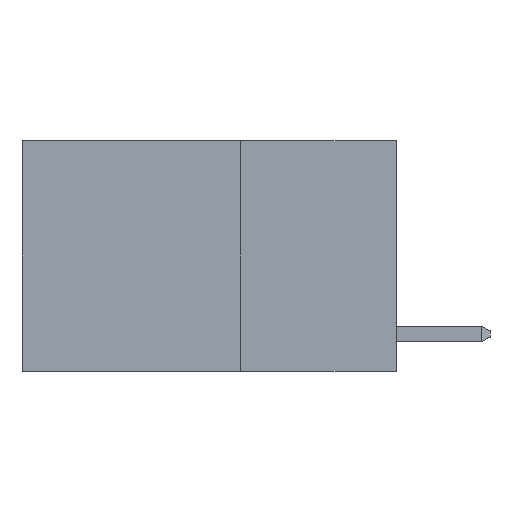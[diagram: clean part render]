
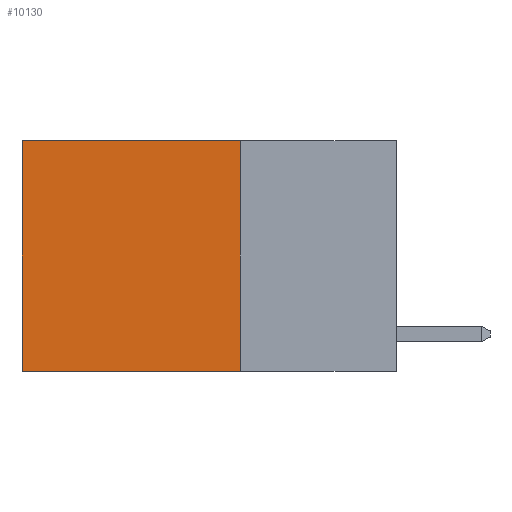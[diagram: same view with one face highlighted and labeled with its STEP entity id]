
A CAD part, left-side view. The second image highlights one B-rep face of the part: STEP entity #10130.
In plain terms, the highlighted planar face has unit normal (-1, 0, 0).
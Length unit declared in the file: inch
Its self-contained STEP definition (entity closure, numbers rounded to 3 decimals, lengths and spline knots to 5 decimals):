
#72 = DIRECTION ( 'NONE',  ( 0., 1., 0. ) ) ;
#144 = AXIS2_PLACEMENT_3D ( 'NONE', #7745, #2744, #8549 ) ;
#897 = VECTOR ( 'NONE', #9569, 39.37008 ) ;
#1374 = LINE ( 'NONE', #5203, #10183 ) ;
#1540 = CARTESIAN_POINT ( 'NONE',  ( 0.2625, 0.25, 0. ) ) ;
#1907 = CARTESIAN_POINT ( 'NONE',  ( 0.2625, 0.6, -0.37 ) ) ;
#2203 = VERTEX_POINT ( 'NONE', #8564 ) ;
#2212 = EDGE_CURVE ( 'NONE', #9869, #2259, #6010, .T. ) ;
#2259 = VERTEX_POINT ( 'NONE', #10237 ) ;
#2744 = DIRECTION ( 'NONE',  ( 1., 0., 0. ) ) ;
#3864 = CARTESIAN_POINT ( 'NONE',  ( 0.2625, 0.25, 0. ) ) ;
#4023 = VECTOR ( 'NONE', #6157, 39.37008 ) ;
#4359 = LINE ( 'NONE', #4698, #897 ) ;
#4404 = PLANE ( 'NONE',  #144 ) ;
#4698 = CARTESIAN_POINT ( 'NONE',  ( 0.2625, 0.6, 0. ) ) ;
#5197 = ORIENTED_EDGE ( 'NONE', *, *, #2212, .T. ) ;
#5203 = CARTESIAN_POINT ( 'NONE',  ( 0.2625, 0.25, -0.37 ) ) ;
#5490 = EDGE_CURVE ( 'NONE', #9869, #2203, #10479, .T. ) ;
#5571 = ORIENTED_EDGE ( 'NONE', *, *, #7923, .F. ) ;
#6010 = LINE ( 'NONE', #10158, #4023 ) ;
#6157 = DIRECTION ( 'NONE',  ( 0., 1., 0. ) ) ;
#6208 = VECTOR ( 'NONE', #8789, 39.37008 ) ;
#6832 = FACE_OUTER_BOUND ( 'NONE', #9192, .T. ) ;
#7659 = ORIENTED_EDGE ( 'NONE', *, *, #9658, .T. ) ;
#7745 = CARTESIAN_POINT ( 'NONE',  ( 0.2625, 0.25, 0. ) ) ;
#7923 = EDGE_CURVE ( 'NONE', #2203, #10164, #1374, .T. ) ;
#8549 = DIRECTION ( 'NONE',  ( 0., 0., -1. ) ) ;
#8564 = CARTESIAN_POINT ( 'NONE',  ( 0.2625, 0.25, -0.37 ) ) ;
#8789 = DIRECTION ( 'NONE',  ( 0., 0., -1. ) ) ;
#9192 = EDGE_LOOP ( 'NONE', ( #7659, #5571, #9690, #5197 ) ) ;
#9569 = DIRECTION ( 'NONE',  ( 0., 0., -1. ) ) ;
#9658 = EDGE_CURVE ( 'NONE', #2259, #10164, #4359, .T. ) ;
#9690 = ORIENTED_EDGE ( 'NONE', *, *, #5490, .F. ) ;
#9869 = VERTEX_POINT ( 'NONE', #1540 ) ;
#10130 = ADVANCED_FACE ( 'NONE', ( #6832 ), #4404, .F. ) ;
#10158 = CARTESIAN_POINT ( 'NONE',  ( 0.2625, 0.25, 0. ) ) ;
#10164 = VERTEX_POINT ( 'NONE', #1907 ) ;
#10183 = VECTOR ( 'NONE', #72, 39.37008 ) ;
#10237 = CARTESIAN_POINT ( 'NONE',  ( 0.2625, 0.6, 0. ) ) ;
#10479 = LINE ( 'NONE', #3864, #6208 ) ;
